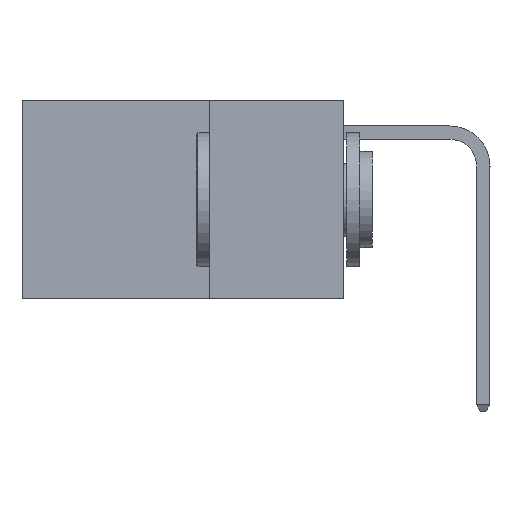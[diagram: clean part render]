
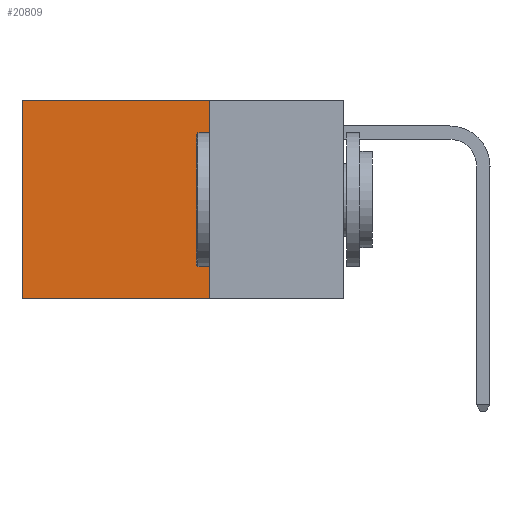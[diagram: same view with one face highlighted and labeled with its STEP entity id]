
A CAD part, left-side view. The second image highlights one B-rep face of the part: STEP entity #20809.
In plain terms, the highlighted planar face has unit normal (-1, 0, 0).
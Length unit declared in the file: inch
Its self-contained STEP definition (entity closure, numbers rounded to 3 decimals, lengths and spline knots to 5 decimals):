
#1387 = EDGE_CURVE ( 'NONE', #3580, #11911, #10895, .T. ) ;
#1493 = CARTESIAN_POINT ( 'NONE',  ( 0.2625, 0.25, 0. ) ) ;
#1558 = DIRECTION ( 'NONE',  ( 0., 1., 0. ) ) ;
#1767 = DIRECTION ( 'NONE',  ( 0., 1., 0. ) ) ;
#2317 = EDGE_CURVE ( 'NONE', #3580, #7137, #14271, .T. ) ;
#2702 = VECTOR ( 'NONE', #1767, 39.37008 ) ;
#3274 = DIRECTION ( 'NONE',  ( 1., 0., 0. ) ) ;
#3331 = CARTESIAN_POINT ( 'NONE',  ( 0.2625, 0.6, 0. ) ) ;
#3580 = VERTEX_POINT ( 'NONE', #11375 ) ;
#4121 = FACE_OUTER_BOUND ( 'NONE', #20632, .T. ) ;
#4635 = ORIENTED_EDGE ( 'NONE', *, *, #16827, .F. ) ;
#5236 = ORIENTED_EDGE ( 'NONE', *, *, #7626, .T. ) ;
#5559 = DIRECTION ( 'NONE',  ( 0., 0., -1. ) ) ;
#6721 = VECTOR ( 'NONE', #5559, 39.37008 ) ;
#7137 = VERTEX_POINT ( 'NONE', #3331 ) ;
#7626 = EDGE_CURVE ( 'NONE', #7137, #15795, #11098, .T. ) ;
#8674 = ORIENTED_EDGE ( 'NONE', *, *, #2317, .T. ) ;
#10487 = CARTESIAN_POINT ( 'NONE',  ( 0.2625, 0.6, 0. ) ) ;
#10895 = LINE ( 'NONE', #19804, #19213 ) ;
#11098 = LINE ( 'NONE', #10487, #6721 ) ;
#11324 = AXIS2_PLACEMENT_3D ( 'NONE', #13253, #3274, #14933 ) ;
#11375 = CARTESIAN_POINT ( 'NONE',  ( 0.2625, 0.25, 0. ) ) ;
#11729 = CARTESIAN_POINT ( 'NONE',  ( 0.2625, 0.25, -0.37 ) ) ;
#11911 = VERTEX_POINT ( 'NONE', #17261 ) ;
#13183 = PLANE ( 'NONE',  #11324 ) ;
#13253 = CARTESIAN_POINT ( 'NONE',  ( 0.2625, 0.25, 0. ) ) ;
#13882 = CARTESIAN_POINT ( 'NONE',  ( 0.2625, 0.6, -0.37 ) ) ;
#14133 = ORIENTED_EDGE ( 'NONE', *, *, #1387, .F. ) ;
#14271 = LINE ( 'NONE', #1493, #18164 ) ;
#14933 = DIRECTION ( 'NONE',  ( 0., 0., -1. ) ) ;
#15479 = LINE ( 'NONE', #11729, #2702 ) ;
#15795 = VERTEX_POINT ( 'NONE', #13882 ) ;
#16827 = EDGE_CURVE ( 'NONE', #11911, #15795, #15479, .T. ) ;
#17261 = CARTESIAN_POINT ( 'NONE',  ( 0.2625, 0.25, -0.37 ) ) ;
#18164 = VECTOR ( 'NONE', #1558, 39.37008 ) ;
#19213 = VECTOR ( 'NONE', #19880, 39.37008 ) ;
#19804 = CARTESIAN_POINT ( 'NONE',  ( 0.2625, 0.25, 0. ) ) ;
#19880 = DIRECTION ( 'NONE',  ( 0., 0., -1. ) ) ;
#20632 = EDGE_LOOP ( 'NONE', ( #5236, #4635, #14133, #8674 ) ) ;
#20809 = ADVANCED_FACE ( 'NONE', ( #4121 ), #13183, .F. ) ;
